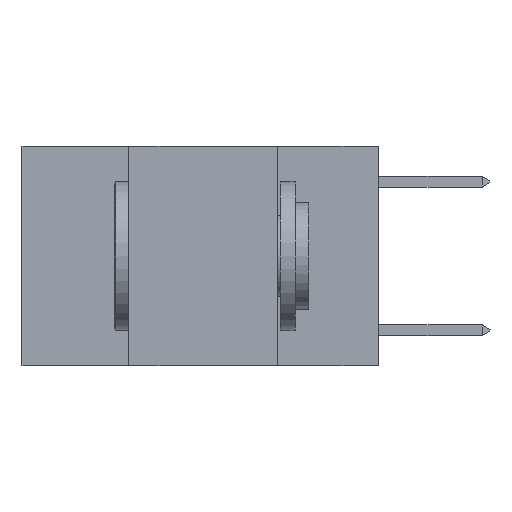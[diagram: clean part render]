
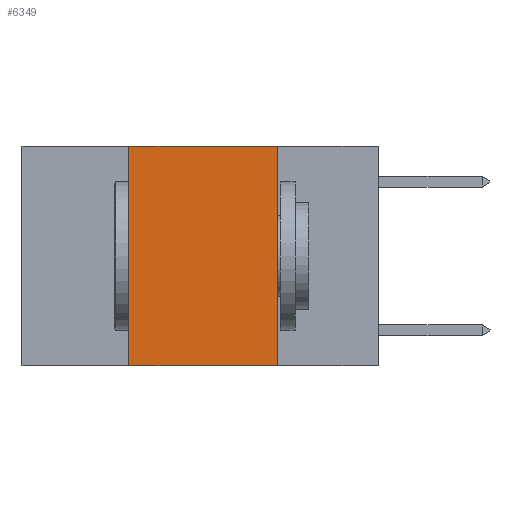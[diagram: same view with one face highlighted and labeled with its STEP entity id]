
A CAD part, left-side view. The second image highlights one B-rep face of the part: STEP entity #6349.
In plain terms, the highlighted planar face has unit normal (-1, 0, 0).
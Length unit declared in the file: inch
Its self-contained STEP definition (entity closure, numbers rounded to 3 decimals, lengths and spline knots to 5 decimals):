
#957 = LINE ( 'NONE', #11462, #15736 ) ;
#1104 = DIRECTION ( 'NONE',  ( 0., -1., 0. ) ) ;
#1488 = LINE ( 'NONE', #5970, #16590 ) ;
#2206 = EDGE_CURVE ( 'NONE', #9894, #11320, #957, .T. ) ;
#2584 = DIRECTION ( 'NONE',  ( 1., 0., 0. ) ) ;
#3048 = CARTESIAN_POINT ( 'NONE',  ( 0., 0.17, -0.37 ) ) ;
#3734 = VECTOR ( 'NONE', #1104, 39.37008 ) ;
#3906 = CARTESIAN_POINT ( 'NONE',  ( 0., 0.6, 0. ) ) ;
#4557 = CARTESIAN_POINT ( 'NONE',  ( 0., 0.6, 0. ) ) ;
#4700 = CARTESIAN_POINT ( 'NONE',  ( 0., 0.17, 0. ) ) ;
#4879 = DIRECTION ( 'NONE',  ( 0., 0., -1. ) ) ;
#5105 = CARTESIAN_POINT ( 'NONE',  ( 0., 0.42, -0.37 ) ) ;
#5970 = CARTESIAN_POINT ( 'NONE',  ( 0., 0.42, 0. ) ) ;
#6349 = ADVANCED_FACE ( 'NONE', ( #6660 ), #10964, .F. ) ;
#6660 = FACE_OUTER_BOUND ( 'NONE', #13804, .T. ) ;
#7393 = DIRECTION ( 'NONE',  ( 0., 0., 1. ) ) ;
#8878 = EDGE_CURVE ( 'NONE', #16148, #11320, #16201, .T. ) ;
#8908 = ORIENTED_EDGE ( 'NONE', *, *, #13630, .F. ) ;
#9894 = VERTEX_POINT ( 'NONE', #5105 ) ;
#9939 = DIRECTION ( 'NONE',  ( 0., -1., 0. ) ) ;
#10299 = ORIENTED_EDGE ( 'NONE', *, *, #8878, .F. ) ;
#10964 = PLANE ( 'NONE',  #16930 ) ;
#11320 = VERTEX_POINT ( 'NONE', #3048 ) ;
#11462 = CARTESIAN_POINT ( 'NONE',  ( 0., 0.6, -0.37 ) ) ;
#11826 = CARTESIAN_POINT ( 'NONE',  ( 0., 0.17, 0. ) ) ;
#13630 = EDGE_CURVE ( 'NONE', #9894, #18022, #1488, .T. ) ;
#13804 = EDGE_LOOP ( 'NONE', ( #10299, #15902, #8908, #14337 ) ) ;
#13963 = DIRECTION ( 'NONE',  ( 0., 0., -1. ) ) ;
#14337 = ORIENTED_EDGE ( 'NONE', *, *, #2206, .T. ) ;
#14720 = LINE ( 'NONE', #4557, #3734 ) ;
#15135 = VECTOR ( 'NONE', #4879, 39.37008 ) ;
#15736 = VECTOR ( 'NONE', #9939, 39.37008 ) ;
#15902 = ORIENTED_EDGE ( 'NONE', *, *, #17548, .F. ) ;
#16148 = VERTEX_POINT ( 'NONE', #11826 ) ;
#16201 = LINE ( 'NONE', #4700, #15135 ) ;
#16235 = CARTESIAN_POINT ( 'NONE',  ( 0., 0.42, 0. ) ) ;
#16590 = VECTOR ( 'NONE', #7393, 39.37008 ) ;
#16930 = AXIS2_PLACEMENT_3D ( 'NONE', #3906, #2584, #13963 ) ;
#17548 = EDGE_CURVE ( 'NONE', #18022, #16148, #14720, .T. ) ;
#18022 = VERTEX_POINT ( 'NONE', #16235 ) ;
